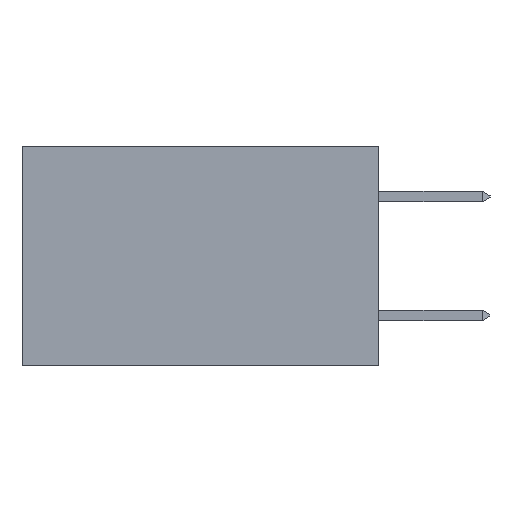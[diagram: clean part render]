
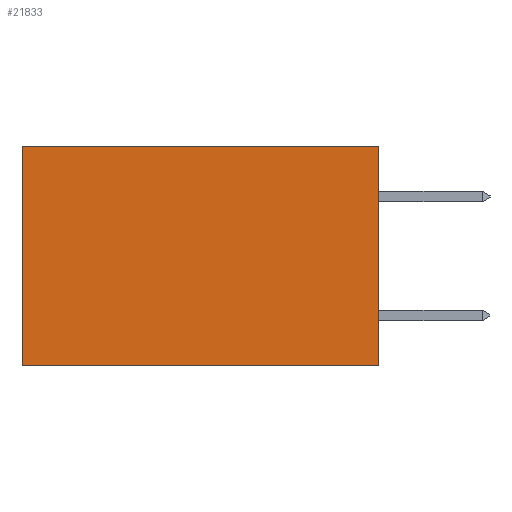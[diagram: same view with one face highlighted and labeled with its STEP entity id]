
A CAD part, left-side view. The second image highlights one B-rep face of the part: STEP entity #21833.
In plain terms, the highlighted planar face has unit normal (-1, 0, 0).
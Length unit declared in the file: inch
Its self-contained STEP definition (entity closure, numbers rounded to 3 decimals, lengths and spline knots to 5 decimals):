
#997 = CARTESIAN_POINT ( 'NONE',  ( 0.298, 0.6, 0. ) ) ;
#1078 = CARTESIAN_POINT ( 'NONE',  ( 0.298, 0., 0. ) ) ;
#1207 = EDGE_CURVE ( 'NONE', #8555, #14033, #20735, .T. ) ;
#2765 = DIRECTION ( 'NONE',  ( 0., 0., -1. ) ) ;
#2855 = DIRECTION ( 'NONE',  ( 0., 0., -1. ) ) ;
#4661 = CARTESIAN_POINT ( 'NONE',  ( 0.298, 0., 0. ) ) ;
#5041 = LINE ( 'NONE', #11643, #8630 ) ;
#5964 = VERTEX_POINT ( 'NONE', #8499 ) ;
#6698 = ORIENTED_EDGE ( 'NONE', *, *, #13849, .T. ) ;
#8085 = PLANE ( 'NONE',  #10454 ) ;
#8298 = CARTESIAN_POINT ( 'NONE',  ( 0.298, 0., -0.37 ) ) ;
#8313 = LINE ( 'NONE', #997, #12986 ) ;
#8462 = CARTESIAN_POINT ( 'NONE',  ( 0.298, 0.6, -0.37 ) ) ;
#8499 = CARTESIAN_POINT ( 'NONE',  ( 0.298, 0.6, 0. ) ) ;
#8555 = VERTEX_POINT ( 'NONE', #8298 ) ;
#8630 = VECTOR ( 'NONE', #20426, 39.37008 ) ;
#9060 = CARTESIAN_POINT ( 'NONE',  ( 0.298, 0., 0. ) ) ;
#9370 = EDGE_LOOP ( 'NONE', ( #6698, #13307, #10210, #13008 ) ) ;
#9950 = LINE ( 'NONE', #9060, #18239 ) ;
#10210 = ORIENTED_EDGE ( 'NONE', *, *, #11817, .F. ) ;
#10454 = AXIS2_PLACEMENT_3D ( 'NONE', #1078, #13397, #2855 ) ;
#10559 = DIRECTION ( 'NONE',  ( 0., 1., 0. ) ) ;
#10838 = DIRECTION ( 'NONE',  ( 0., 1., 0. ) ) ;
#11643 = CARTESIAN_POINT ( 'NONE',  ( 0.298, 0., 0. ) ) ;
#11817 = EDGE_CURVE ( 'NONE', #18862, #8555, #5041, .T. ) ;
#12986 = VECTOR ( 'NONE', #2765, 39.37008 ) ;
#13008 = ORIENTED_EDGE ( 'NONE', *, *, #14254, .T. ) ;
#13307 = ORIENTED_EDGE ( 'NONE', *, *, #1207, .F. ) ;
#13397 = DIRECTION ( 'NONE',  ( 1., 0., 0. ) ) ;
#13849 = EDGE_CURVE ( 'NONE', #5964, #14033, #8313, .T. ) ;
#14033 = VERTEX_POINT ( 'NONE', #8462 ) ;
#14254 = EDGE_CURVE ( 'NONE', #18862, #5964, #9950, .T. ) ;
#16196 = CARTESIAN_POINT ( 'NONE',  ( 0.298, 0., -0.37 ) ) ;
#16626 = FACE_OUTER_BOUND ( 'NONE', #9370, .T. ) ;
#18239 = VECTOR ( 'NONE', #10838, 39.37008 ) ;
#18862 = VERTEX_POINT ( 'NONE', #4661 ) ;
#20190 = VECTOR ( 'NONE', #10559, 39.37008 ) ;
#20426 = DIRECTION ( 'NONE',  ( 0., 0., -1. ) ) ;
#20735 = LINE ( 'NONE', #16196, #20190 ) ;
#21833 = ADVANCED_FACE ( 'NONE', ( #16626 ), #8085, .F. ) ;
